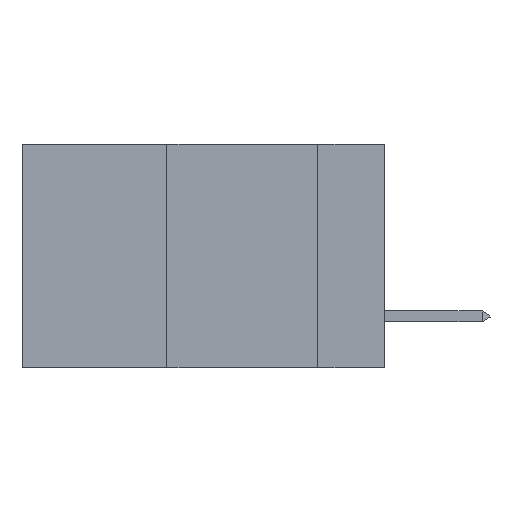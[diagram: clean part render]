
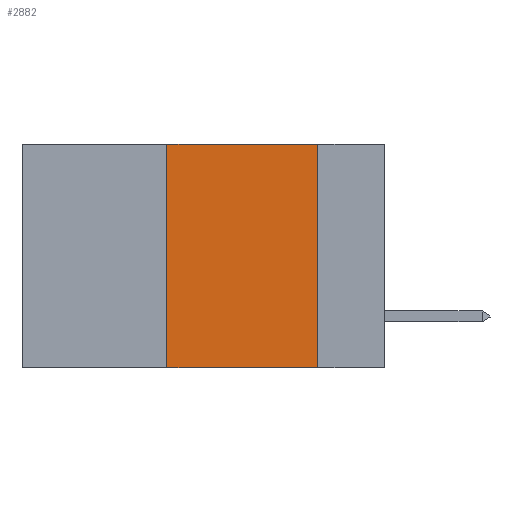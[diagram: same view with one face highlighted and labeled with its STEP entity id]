
A CAD part, left-side view. The second image highlights one B-rep face of the part: STEP entity #2882.
In plain terms, the highlighted planar face has unit normal (-1, 0, 0).
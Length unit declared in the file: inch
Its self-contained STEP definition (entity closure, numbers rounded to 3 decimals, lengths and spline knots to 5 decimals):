
#601 = VECTOR ( 'NONE', #9966, 39.37008 ) ;
#1038 = CARTESIAN_POINT ( 'NONE',  ( 0., 0.36, 0. ) ) ;
#1643 = CARTESIAN_POINT ( 'NONE',  ( 0., 0.6, 0. ) ) ;
#2882 = ADVANCED_FACE ( 'NONE', ( #31547 ), #3284, .F. ) ;
#3143 = DIRECTION ( 'NONE',  ( 1., 0., 0. ) ) ;
#3284 = PLANE ( 'NONE',  #10631 ) ;
#6637 = ORIENTED_EDGE ( 'NONE', *, *, #26361, .F. ) ;
#7249 = CARTESIAN_POINT ( 'NONE',  ( 0., 0.11, -0.37 ) ) ;
#7342 = CARTESIAN_POINT ( 'NONE',  ( 0., 0.6, -0.37 ) ) ;
#8061 = VERTEX_POINT ( 'NONE', #7249 ) ;
#9966 = DIRECTION ( 'NONE',  ( 0., 0., 1. ) ) ;
#10451 = EDGE_CURVE ( 'NONE', #16975, #34459, #36834, .T. ) ;
#10631 = AXIS2_PLACEMENT_3D ( 'NONE', #21889, #3143, #34492 ) ;
#10873 = LINE ( 'NONE', #7342, #29168 ) ;
#12893 = CARTESIAN_POINT ( 'NONE',  ( 0., 0.36, 0. ) ) ;
#13281 = EDGE_CURVE ( 'NONE', #34459, #15868, #28273, .T. ) ;
#13764 = DIRECTION ( 'NONE',  ( 0., -1., 0. ) ) ;
#14117 = LINE ( 'NONE', #20437, #18572 ) ;
#15868 = VERTEX_POINT ( 'NONE', #26318 ) ;
#16957 = ORIENTED_EDGE ( 'NONE', *, *, #13281, .F. ) ;
#16975 = VERTEX_POINT ( 'NONE', #24917 ) ;
#17454 = VECTOR ( 'NONE', #13764, 39.37008 ) ;
#18572 = VECTOR ( 'NONE', #26947, 39.37008 ) ;
#20437 = CARTESIAN_POINT ( 'NONE',  ( 0., 0.11, 0. ) ) ;
#21889 = CARTESIAN_POINT ( 'NONE',  ( 0., 0.6, 0. ) ) ;
#23834 = EDGE_CURVE ( 'NONE', #16975, #8061, #10873, .T. ) ;
#24917 = CARTESIAN_POINT ( 'NONE',  ( 0., 0.36, -0.37 ) ) ;
#26318 = CARTESIAN_POINT ( 'NONE',  ( 0., 0.11, 0. ) ) ;
#26361 = EDGE_CURVE ( 'NONE', #15868, #8061, #14117, .T. ) ;
#26947 = DIRECTION ( 'NONE',  ( 0., 0., -1. ) ) ;
#28273 = LINE ( 'NONE', #1643, #17454 ) ;
#29168 = VECTOR ( 'NONE', #39064, 39.37008 ) ;
#30189 = ORIENTED_EDGE ( 'NONE', *, *, #23834, .T. ) ;
#31281 = EDGE_LOOP ( 'NONE', ( #6637, #16957, #34293, #30189 ) ) ;
#31547 = FACE_OUTER_BOUND ( 'NONE', #31281, .T. ) ;
#34293 = ORIENTED_EDGE ( 'NONE', *, *, #10451, .F. ) ;
#34459 = VERTEX_POINT ( 'NONE', #1038 ) ;
#34492 = DIRECTION ( 'NONE',  ( 0., 0., -1. ) ) ;
#36834 = LINE ( 'NONE', #12893, #601 ) ;
#39064 = DIRECTION ( 'NONE',  ( 0., -1., 0. ) ) ;
